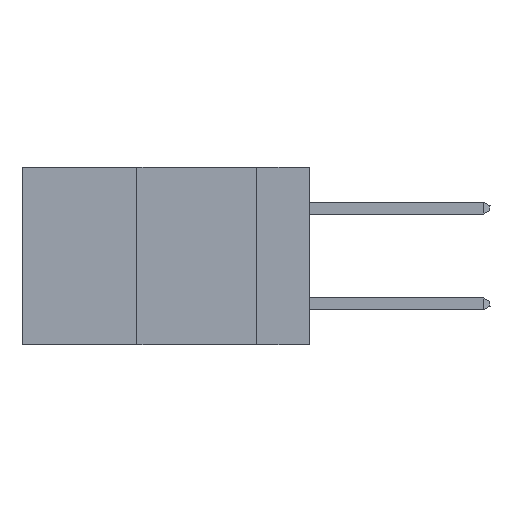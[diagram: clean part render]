
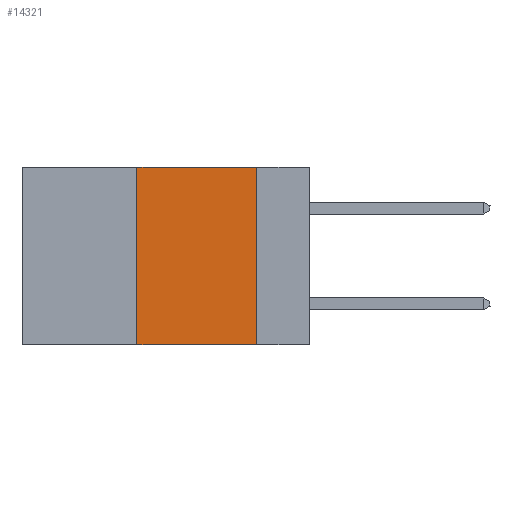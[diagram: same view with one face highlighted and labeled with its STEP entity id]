
A CAD part, left-side view. The second image highlights one B-rep face of the part: STEP entity #14321.
In plain terms, the highlighted planar face has unit normal (-1, 0, 0).
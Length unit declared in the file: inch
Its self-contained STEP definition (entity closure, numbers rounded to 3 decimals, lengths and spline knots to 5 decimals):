
#1325 = LINE ( 'NONE', #22587, #19525 ) ;
#2185 = CARTESIAN_POINT ( 'NONE',  ( 0., 0.11, 0. ) ) ;
#2398 = VERTEX_POINT ( 'NONE', #8330 ) ;
#3032 = DIRECTION ( 'NONE',  ( 1., 0., 0. ) ) ;
#3686 = DIRECTION ( 'NONE',  ( 0., 0., -1. ) ) ;
#4201 = ORIENTED_EDGE ( 'NONE', *, *, #27076, .T. ) ;
#4656 = CARTESIAN_POINT ( 'NONE',  ( 0., 0.36, -0.37 ) ) ;
#4846 = CARTESIAN_POINT ( 'NONE',  ( 0., 0.36, 0. ) ) ;
#5922 = LINE ( 'NONE', #11085, #29010 ) ;
#7969 = VERTEX_POINT ( 'NONE', #18674 ) ;
#8330 = CARTESIAN_POINT ( 'NONE',  ( 0., 0.36, 0. ) ) ;
#8899 = VERTEX_POINT ( 'NONE', #4656 ) ;
#9007 = DIRECTION ( 'NONE',  ( 0., -1., 0. ) ) ;
#10306 = DIRECTION ( 'NONE',  ( 0., -1., 0. ) ) ;
#10430 = EDGE_LOOP ( 'NONE', ( #31498, #28867, #14283, #4201 ) ) ;
#10528 = EDGE_CURVE ( 'NONE', #21844, #7969, #5922, .T. ) ;
#11085 = CARTESIAN_POINT ( 'NONE',  ( 0., 0.11, 0. ) ) ;
#12197 = FACE_OUTER_BOUND ( 'NONE', #10430, .T. ) ;
#12455 = AXIS2_PLACEMENT_3D ( 'NONE', #17872, #3032, #20328 ) ;
#12464 = VECTOR ( 'NONE', #9007, 39.37008 ) ;
#14283 = ORIENTED_EDGE ( 'NONE', *, *, #29661, .F. ) ;
#14289 = EDGE_CURVE ( 'NONE', #2398, #21844, #1325, .T. ) ;
#14321 = ADVANCED_FACE ( 'NONE', ( #12197 ), #30028, .F. ) ;
#17872 = CARTESIAN_POINT ( 'NONE',  ( 0., 0.6, 0. ) ) ;
#18674 = CARTESIAN_POINT ( 'NONE',  ( 0., 0.11, -0.37 ) ) ;
#19525 = VECTOR ( 'NONE', #10306, 39.37008 ) ;
#19676 = DIRECTION ( 'NONE',  ( 0., 0., 1. ) ) ;
#20328 = DIRECTION ( 'NONE',  ( 0., 0., -1. ) ) ;
#21844 = VERTEX_POINT ( 'NONE', #2185 ) ;
#22587 = CARTESIAN_POINT ( 'NONE',  ( 0., 0.6, 0. ) ) ;
#23776 = CARTESIAN_POINT ( 'NONE',  ( 0., 0.6, -0.37 ) ) ;
#25515 = LINE ( 'NONE', #23776, #12464 ) ;
#27076 = EDGE_CURVE ( 'NONE', #8899, #7969, #25515, .T. ) ;
#27625 = VECTOR ( 'NONE', #19676, 39.37008 ) ;
#28388 = LINE ( 'NONE', #4846, #27625 ) ;
#28867 = ORIENTED_EDGE ( 'NONE', *, *, #14289, .F. ) ;
#29010 = VECTOR ( 'NONE', #3686, 39.37008 ) ;
#29661 = EDGE_CURVE ( 'NONE', #8899, #2398, #28388, .T. ) ;
#30028 = PLANE ( 'NONE',  #12455 ) ;
#31498 = ORIENTED_EDGE ( 'NONE', *, *, #10528, .F. ) ;
